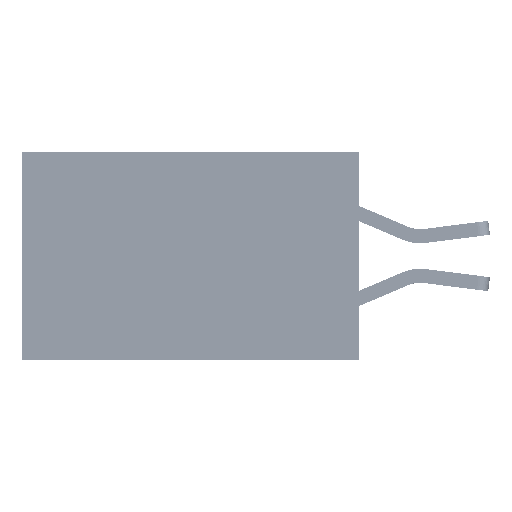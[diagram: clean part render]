
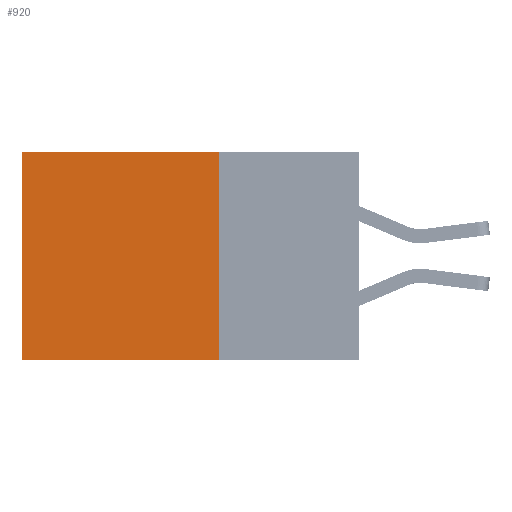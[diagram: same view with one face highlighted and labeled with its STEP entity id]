
A CAD part, left-side view. The second image highlights one B-rep face of the part: STEP entity #920.
In plain terms, the highlighted planar face has unit normal (-1, 0, 0).
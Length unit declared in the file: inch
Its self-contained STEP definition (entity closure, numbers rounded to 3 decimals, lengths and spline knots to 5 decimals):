
#920 = ADVANCED_FACE ( 'NONE', ( #7782 ), #4889, .F. ) ;
#3555 = CARTESIAN_POINT ( 'NONE',  ( 0.2875, 0.25, 0. ) ) ;
#4090 = DIRECTION ( 'NONE',  ( 0., 1., 0. ) ) ;
#4650 = ORIENTED_EDGE ( 'NONE', *, *, #22595, .T. ) ;
#4856 = AXIS2_PLACEMENT_3D ( 'NONE', #37067, #8130, #14331 ) ;
#4889 = PLANE ( 'NONE',  #4856 ) ;
#5472 = VERTEX_POINT ( 'NONE', #40449 ) ;
#7045 = CARTESIAN_POINT ( 'NONE',  ( 0.2875, 0.25, 0. ) ) ;
#7782 = FACE_OUTER_BOUND ( 'NONE', #21833, .T. ) ;
#8130 = DIRECTION ( 'NONE',  ( 1., 0., 0. ) ) ;
#8669 = EDGE_CURVE ( 'NONE', #5472, #8905, #9938, .T. ) ;
#8905 = VERTEX_POINT ( 'NONE', #31254 ) ;
#9183 = EDGE_CURVE ( 'NONE', #37558, #35608, #10896, .T. ) ;
#9875 = LINE ( 'NONE', #16093, #32188 ) ;
#9938 = LINE ( 'NONE', #20552, #23651 ) ;
#10896 = LINE ( 'NONE', #3555, #12379 ) ;
#12379 = VECTOR ( 'NONE', #26117, 39.37008 ) ;
#13190 = ORIENTED_EDGE ( 'NONE', *, *, #16623, .F. ) ;
#14331 = DIRECTION ( 'NONE',  ( 0., 0., -1. ) ) ;
#14475 = VECTOR ( 'NONE', #4090, 39.37008 ) ;
#16093 = CARTESIAN_POINT ( 'NONE',  ( 0.2875, 0.25, -0.37 ) ) ;
#16202 = ORIENTED_EDGE ( 'NONE', *, *, #8669, .T. ) ;
#16267 = CARTESIAN_POINT ( 'NONE',  ( 0.2875, 0.25, -0.37 ) ) ;
#16623 = EDGE_CURVE ( 'NONE', #35608, #8905, #9875, .T. ) ;
#20552 = CARTESIAN_POINT ( 'NONE',  ( 0.2875, 0.6, 0. ) ) ;
#21833 = EDGE_LOOP ( 'NONE', ( #16202, #13190, #35045, #4650 ) ) ;
#22595 = EDGE_CURVE ( 'NONE', #37558, #5472, #40203, .T. ) ;
#23651 = VECTOR ( 'NONE', #26995, 39.37008 ) ;
#25834 = DIRECTION ( 'NONE',  ( 0., 1., 0. ) ) ;
#26117 = DIRECTION ( 'NONE',  ( 0., 0., -1. ) ) ;
#26995 = DIRECTION ( 'NONE',  ( 0., 0., -1. ) ) ;
#31254 = CARTESIAN_POINT ( 'NONE',  ( 0.2875, 0.6, -0.37 ) ) ;
#32188 = VECTOR ( 'NONE', #25834, 39.37008 ) ;
#35045 = ORIENTED_EDGE ( 'NONE', *, *, #9183, .F. ) ;
#35608 = VERTEX_POINT ( 'NONE', #16267 ) ;
#37067 = CARTESIAN_POINT ( 'NONE',  ( 0.2875, 0.25, 0. ) ) ;
#37091 = CARTESIAN_POINT ( 'NONE',  ( 0.2875, 0.25, 0. ) ) ;
#37558 = VERTEX_POINT ( 'NONE', #37091 ) ;
#40203 = LINE ( 'NONE', #7045, #14475 ) ;
#40449 = CARTESIAN_POINT ( 'NONE',  ( 0.2875, 0.6, 0. ) ) ;
